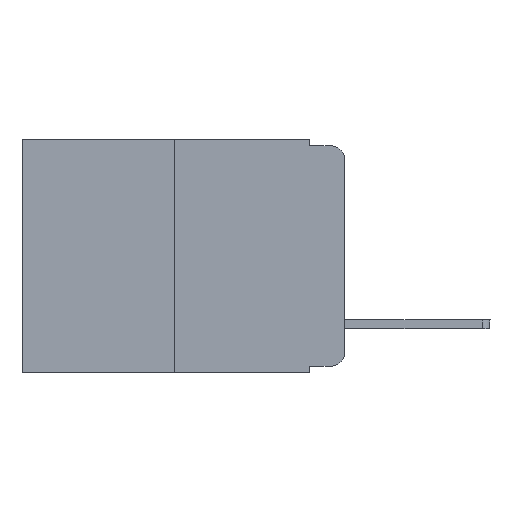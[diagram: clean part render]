
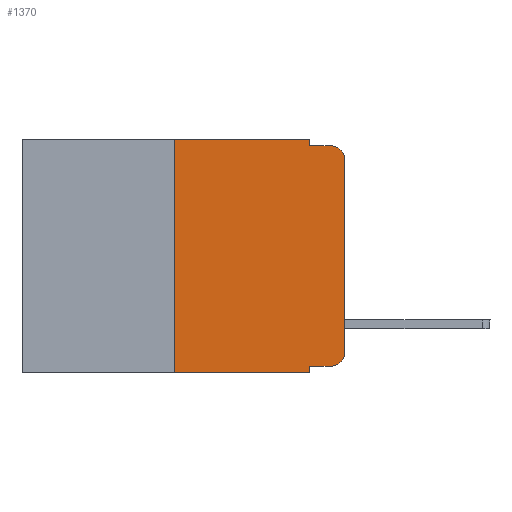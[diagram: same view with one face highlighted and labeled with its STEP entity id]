
A CAD part, left-side view. The second image highlights one B-rep face of the part: STEP entity #1370.
In plain terms, the highlighted planar face has unit normal (-1, 0, 0).
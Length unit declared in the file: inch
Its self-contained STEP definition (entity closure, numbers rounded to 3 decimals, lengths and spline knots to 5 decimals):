
#99 = ORIENTED_EDGE ( 'NONE', *, *, #9783, .T. ) ;
#153 = DIRECTION ( 'NONE',  ( 1., 0., 0. ) ) ;
#159 = LINE ( 'NONE', #3269, #4730 ) ;
#241 = VERTEX_POINT ( 'NONE', #5330 ) ;
#473 = DIRECTION ( 'NONE',  ( 0., -1., 0. ) ) ;
#817 = CARTESIAN_POINT ( 'NONE',  ( 0., 0.25, 0. ) ) ;
#1260 = ORIENTED_EDGE ( 'NONE', *, *, #12436, .T. ) ;
#1370 = ADVANCED_FACE ( 'NONE', ( #4059 ), #10116, .F. ) ;
#1453 = VECTOR ( 'NONE', #4329, 39.37008 ) ;
#1976 = DIRECTION ( 'NONE',  ( 0., 0., 1. ) ) ;
#2125 = DIRECTION ( 'NONE',  ( 0., 0., -1. ) ) ;
#2403 = LINE ( 'NONE', #6539, #3874 ) ;
#2584 = CARTESIAN_POINT ( 'NONE',  ( 0., 0., -0.313 ) ) ;
#2771 = VERTEX_POINT ( 'NONE', #9450 ) ;
#3134 = CARTESIAN_POINT ( 'NONE',  ( 0., 0.02, -0.313 ) ) ;
#3189 = EDGE_CURVE ( 'NONE', #8144, #8233, #8786, .T. ) ;
#3214 = DIRECTION ( 'NONE',  ( 0., 0., 1. ) ) ;
#3255 = VECTOR ( 'NONE', #1976, 39.37008 ) ;
#3269 = CARTESIAN_POINT ( 'NONE',  ( 0., 0.473, 0. ) ) ;
#3399 = CARTESIAN_POINT ( 'NONE',  ( 0., 0.473, -0.343 ) ) ;
#3722 = DIRECTION ( 'NONE',  ( 0., -1., 0. ) ) ;
#3874 = VECTOR ( 'NONE', #3214, 39.37008 ) ;
#3944 = DIRECTION ( 'NONE',  ( 0., 0., -1. ) ) ;
#4057 = ORIENTED_EDGE ( 'NONE', *, *, #8187, .T. ) ;
#4059 = FACE_OUTER_BOUND ( 'NONE', #12003, .T. ) ;
#4152 = EDGE_CURVE ( 'NONE', #2771, #7827, #5627, .T. ) ;
#4181 = VERTEX_POINT ( 'NONE', #7691 ) ;
#4289 = AXIS2_PLACEMENT_3D ( 'NONE', #11316, #153, #2125 ) ;
#4290 = ORIENTED_EDGE ( 'NONE', *, *, #3189, .T. ) ;
#4329 = DIRECTION ( 'NONE',  ( 0., -1., 0. ) ) ;
#4368 = EDGE_CURVE ( 'NONE', #241, #4181, #10129, .T. ) ;
#4730 = VECTOR ( 'NONE', #473, 39.37008 ) ;
#4735 = VERTEX_POINT ( 'NONE', #10988 ) ;
#4747 = AXIS2_PLACEMENT_3D ( 'NONE', #3134, #7217, #10262 ) ;
#4806 = ORIENTED_EDGE ( 'NONE', *, *, #4152, .F. ) ;
#4807 = CARTESIAN_POINT ( 'NONE',  ( 0., 0.051, 0. ) ) ;
#5308 = CIRCLE ( 'NONE', #11468, 0.02 ) ;
#5330 = CARTESIAN_POINT ( 'NONE',  ( 0., 0.051, -0.333 ) ) ;
#5627 = LINE ( 'NONE', #10883, #9410 ) ;
#5713 = ORIENTED_EDGE ( 'NONE', *, *, #9092, .F. ) ;
#5745 = CARTESIAN_POINT ( 'NONE',  ( 0., 0.02, -0.01 ) ) ;
#6034 = VERTEX_POINT ( 'NONE', #6198 ) ;
#6157 = EDGE_CURVE ( 'NONE', #241, #8144, #11846, .T. ) ;
#6198 = CARTESIAN_POINT ( 'NONE',  ( 0., 0.25, -0.343 ) ) ;
#6539 = CARTESIAN_POINT ( 'NONE',  ( 0., 0.25, 0. ) ) ;
#7196 = DIRECTION ( 'NONE',  ( 0., 0., -1. ) ) ;
#7217 = DIRECTION ( 'NONE',  ( -1., 0., 0. ) ) ;
#7594 = CARTESIAN_POINT ( 'NONE',  ( 0., 0.051, -0.333 ) ) ;
#7691 = CARTESIAN_POINT ( 'NONE',  ( 0., 0.051, -0.343 ) ) ;
#7779 = ORIENTED_EDGE ( 'NONE', *, *, #11724, .F. ) ;
#7827 = VERTEX_POINT ( 'NONE', #5745 ) ;
#8144 = VERTEX_POINT ( 'NONE', #11719 ) ;
#8187 = EDGE_CURVE ( 'NONE', #6034, #4181, #9387, .T. ) ;
#8233 = VERTEX_POINT ( 'NONE', #2584 ) ;
#8320 = DIRECTION ( 'NONE',  ( -1., 0., 0. ) ) ;
#8786 = CIRCLE ( 'NONE', #4747, 0.02 ) ;
#8949 = VERTEX_POINT ( 'NONE', #817 ) ;
#9092 = EDGE_CURVE ( 'NONE', #4735, #2771, #10669, .T. ) ;
#9225 = LINE ( 'NONE', #10224, #3255 ) ;
#9387 = LINE ( 'NONE', #3399, #1453 ) ;
#9410 = VECTOR ( 'NONE', #9670, 39.37008 ) ;
#9450 = CARTESIAN_POINT ( 'NONE',  ( 0., 0.051, -0.01 ) ) ;
#9664 = DIRECTION ( 'NONE',  ( 0., 0., -1. ) ) ;
#9670 = DIRECTION ( 'NONE',  ( 0., -1., 0. ) ) ;
#9737 = VECTOR ( 'NONE', #9664, 39.37008 ) ;
#9783 = EDGE_CURVE ( 'NONE', #12621, #7827, #5308, .T. ) ;
#10116 = PLANE ( 'NONE',  #4289 ) ;
#10129 = LINE ( 'NONE', #4807, #12616 ) ;
#10224 = CARTESIAN_POINT ( 'NONE',  ( 0., 0., 0. ) ) ;
#10262 = DIRECTION ( 'NONE',  ( 0., 0., -1. ) ) ;
#10565 = ORIENTED_EDGE ( 'NONE', *, *, #12160, .F. ) ;
#10669 = LINE ( 'NONE', #12742, #9737 ) ;
#10883 = CARTESIAN_POINT ( 'NONE',  ( 0., 0.051, -0.01 ) ) ;
#10988 = CARTESIAN_POINT ( 'NONE',  ( 0., 0.051, 0. ) ) ;
#11316 = CARTESIAN_POINT ( 'NONE',  ( 0., 0.473, 0. ) ) ;
#11468 = AXIS2_PLACEMENT_3D ( 'NONE', #12248, #8320, #7196 ) ;
#11719 = CARTESIAN_POINT ( 'NONE',  ( 0., 0.02, -0.333 ) ) ;
#11724 = EDGE_CURVE ( 'NONE', #6034, #8949, #2403, .T. ) ;
#11846 = LINE ( 'NONE', #7594, #12308 ) ;
#12003 = EDGE_LOOP ( 'NONE', ( #1260, #99, #4806, #5713, #10565, #7779, #4057, #12287, #13007, #4290 ) ) ;
#12020 = CARTESIAN_POINT ( 'NONE',  ( 0., 0., -0.03 ) ) ;
#12160 = EDGE_CURVE ( 'NONE', #8949, #4735, #159, .T. ) ;
#12248 = CARTESIAN_POINT ( 'NONE',  ( 0., 0.02, -0.03 ) ) ;
#12287 = ORIENTED_EDGE ( 'NONE', *, *, #4368, .F. ) ;
#12308 = VECTOR ( 'NONE', #3722, 39.37008 ) ;
#12436 = EDGE_CURVE ( 'NONE', #8233, #12621, #9225, .T. ) ;
#12616 = VECTOR ( 'NONE', #3944, 39.37008 ) ;
#12621 = VERTEX_POINT ( 'NONE', #12020 ) ;
#12742 = CARTESIAN_POINT ( 'NONE',  ( 0., 0.051, 0. ) ) ;
#13007 = ORIENTED_EDGE ( 'NONE', *, *, #6157, .T. ) ;
